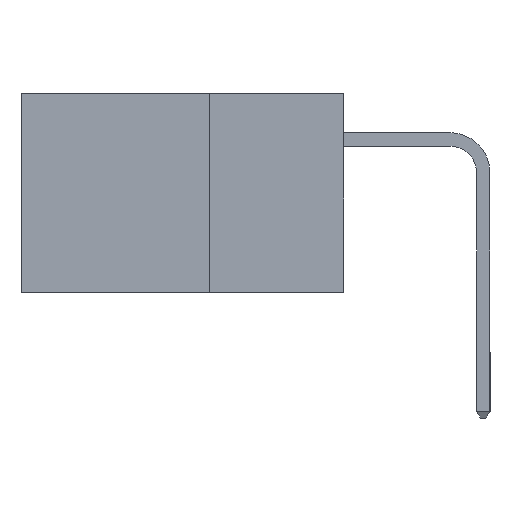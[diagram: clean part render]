
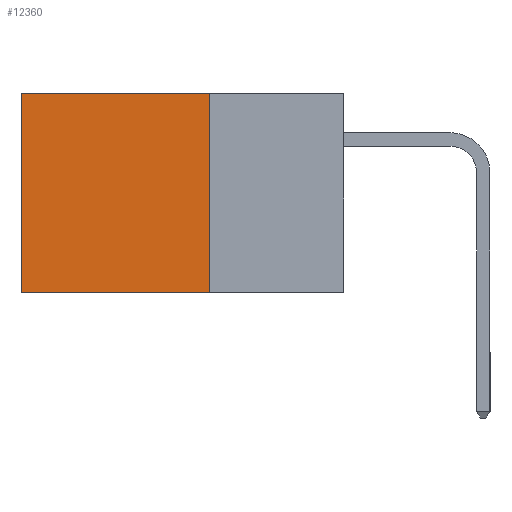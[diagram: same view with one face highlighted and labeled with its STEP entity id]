
A CAD part, left-side view. The second image highlights one B-rep face of the part: STEP entity #12360.
In plain terms, the highlighted planar face has unit normal (-1, 0, 0).
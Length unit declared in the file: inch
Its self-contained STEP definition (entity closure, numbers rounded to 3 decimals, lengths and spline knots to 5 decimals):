
#108 = DIRECTION ( 'NONE',  ( 0., 0., -1. ) ) ;
#209 = VERTEX_POINT ( 'NONE', #2833 ) ;
#1102 = CARTESIAN_POINT ( 'NONE',  ( 0.298, 0.25, 0. ) ) ;
#1769 = ORIENTED_EDGE ( 'NONE', *, *, #5438, .F. ) ;
#2086 = VECTOR ( 'NONE', #18362, 39.37008 ) ;
#2463 = AXIS2_PLACEMENT_3D ( 'NONE', #4800, #10982, #6122 ) ;
#2833 = CARTESIAN_POINT ( 'NONE',  ( 0.298, 0.6, -0.37 ) ) ;
#3925 = CARTESIAN_POINT ( 'NONE',  ( 0.298, 0.6, 0. ) ) ;
#4183 = LINE ( 'NONE', #18487, #2086 ) ;
#4687 = VERTEX_POINT ( 'NONE', #6296 ) ;
#4800 = CARTESIAN_POINT ( 'NONE',  ( 0.298, 0.25, 0. ) ) ;
#5061 = ORIENTED_EDGE ( 'NONE', *, *, #18922, .T. ) ;
#5438 = EDGE_CURVE ( 'NONE', #4687, #15582, #11122, .T. ) ;
#6122 = DIRECTION ( 'NONE',  ( 0., 0., -1. ) ) ;
#6269 = VECTOR ( 'NONE', #6918, 39.37008 ) ;
#6296 = CARTESIAN_POINT ( 'NONE',  ( 0.298, 0.25, 0. ) ) ;
#6859 = VECTOR ( 'NONE', #108, 39.37008 ) ;
#6918 = DIRECTION ( 'NONE',  ( 0., 1., 0. ) ) ;
#7360 = VECTOR ( 'NONE', #9748, 39.37008 ) ;
#7760 = CARTESIAN_POINT ( 'NONE',  ( 0.298, 0.6, 0. ) ) ;
#9439 = PLANE ( 'NONE',  #2463 ) ;
#9748 = DIRECTION ( 'NONE',  ( 0., 0., -1. ) ) ;
#10025 = CARTESIAN_POINT ( 'NONE',  ( 0.298, 0.25, -0.37 ) ) ;
#10670 = ORIENTED_EDGE ( 'NONE', *, *, #18022, .F. ) ;
#10672 = FACE_OUTER_BOUND ( 'NONE', #15300, .T. ) ;
#10982 = DIRECTION ( 'NONE',  ( 1., 0., 0. ) ) ;
#11122 = LINE ( 'NONE', #16250, #6859 ) ;
#11150 = LINE ( 'NONE', #3925, #7360 ) ;
#12360 = ADVANCED_FACE ( 'NONE', ( #10672 ), #9439, .F. ) ;
#14737 = VERTEX_POINT ( 'NONE', #7760 ) ;
#15300 = EDGE_LOOP ( 'NONE', ( #16554, #10670, #1769, #5061 ) ) ;
#15582 = VERTEX_POINT ( 'NONE', #10025 ) ;
#15938 = EDGE_CURVE ( 'NONE', #14737, #209, #11150, .T. ) ;
#16250 = CARTESIAN_POINT ( 'NONE',  ( 0.298, 0.25, 0. ) ) ;
#16554 = ORIENTED_EDGE ( 'NONE', *, *, #15938, .T. ) ;
#18022 = EDGE_CURVE ( 'NONE', #15582, #209, #4183, .T. ) ;
#18362 = DIRECTION ( 'NONE',  ( 0., 1., 0. ) ) ;
#18452 = LINE ( 'NONE', #1102, #6269 ) ;
#18487 = CARTESIAN_POINT ( 'NONE',  ( 0.298, 0.25, -0.37 ) ) ;
#18922 = EDGE_CURVE ( 'NONE', #4687, #14737, #18452, .T. ) ;
